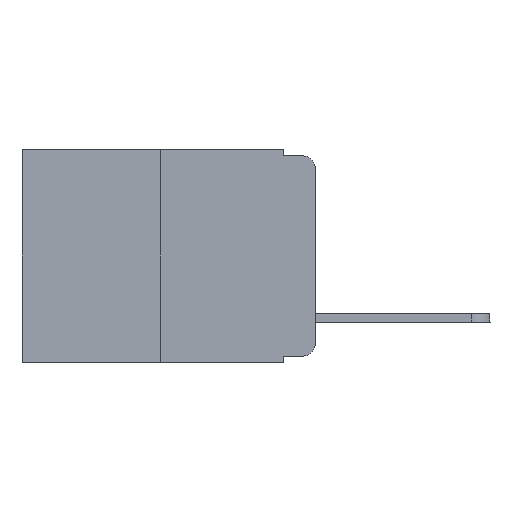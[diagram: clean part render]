
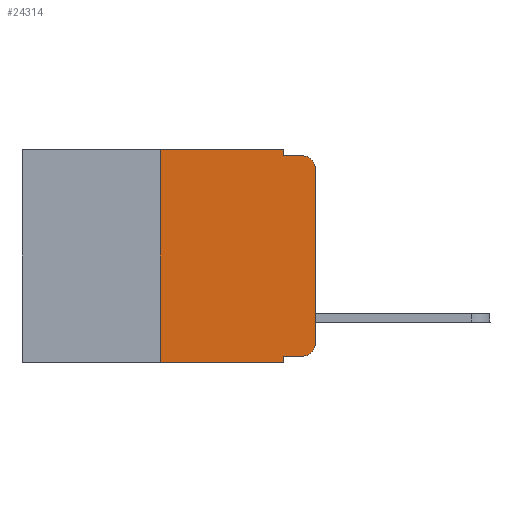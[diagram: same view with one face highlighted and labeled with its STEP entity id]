
A CAD part, left-side view. The second image highlights one B-rep face of the part: STEP entity #24314.
In plain terms, the highlighted planar face has unit normal (-1, 0, 0).
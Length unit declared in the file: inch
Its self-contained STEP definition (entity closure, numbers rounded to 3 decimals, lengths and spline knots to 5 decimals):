
#302 = VECTOR ( 'NONE', #13397, 39.37008 ) ;
#645 = CARTESIAN_POINT ( 'NONE',  ( 0., 0.473, 0. ) ) ;
#865 = ORIENTED_EDGE ( 'NONE', *, *, #11124, .T. ) ;
#1724 = DIRECTION ( 'NONE',  ( -1., 0., 0. ) ) ;
#1776 = VERTEX_POINT ( 'NONE', #15486 ) ;
#2022 = EDGE_CURVE ( 'NONE', #14431, #3511, #22727, .T. ) ;
#2153 = AXIS2_PLACEMENT_3D ( 'NONE', #15584, #1724, #21444 ) ;
#2289 = DIRECTION ( 'NONE',  ( 0., 0., -1. ) ) ;
#2413 = CARTESIAN_POINT ( 'NONE',  ( 0., 0., -0.03 ) ) ;
#2669 = EDGE_CURVE ( 'NONE', #3511, #21373, #8238, .T. ) ;
#3124 = EDGE_CURVE ( 'NONE', #24070, #15990, #22677, .T. ) ;
#3193 = CARTESIAN_POINT ( 'NONE',  ( 0., 0.051, 0. ) ) ;
#3511 = VERTEX_POINT ( 'NONE', #5101 ) ;
#3646 = LINE ( 'NONE', #9644, #7637 ) ;
#3664 = CIRCLE ( 'NONE', #4204, 0.02 ) ;
#3833 = VECTOR ( 'NONE', #7618, 39.37008 ) ;
#4204 = AXIS2_PLACEMENT_3D ( 'NONE', #8919, #16780, #22647 ) ;
#5101 = CARTESIAN_POINT ( 'NONE',  ( 0., 0.051, -0.01 ) ) ;
#5579 = ORIENTED_EDGE ( 'NONE', *, *, #6956, .F. ) ;
#6323 = VECTOR ( 'NONE', #7011, 39.37008 ) ;
#6493 = DIRECTION ( 'NONE',  ( 0., -1., 0. ) ) ;
#6956 = EDGE_CURVE ( 'NONE', #12416, #1776, #3646, .T. ) ;
#7011 = DIRECTION ( 'NONE',  ( 0., 0., 1. ) ) ;
#7618 = DIRECTION ( 'NONE',  ( 0., 0., -1. ) ) ;
#7637 = VECTOR ( 'NONE', #7837, 39.37008 ) ;
#7803 = DIRECTION ( 'NONE',  ( 1., 0., 0. ) ) ;
#7837 = DIRECTION ( 'NONE',  ( 0., 0., 1. ) ) ;
#8234 = ORIENTED_EDGE ( 'NONE', *, *, #22023, .T. ) ;
#8238 = LINE ( 'NONE', #8549, #23303 ) ;
#8549 = CARTESIAN_POINT ( 'NONE',  ( 0., 0.051, -0.01 ) ) ;
#8795 = DIRECTION ( 'NONE',  ( 0., -1., 0. ) ) ;
#8837 = ORIENTED_EDGE ( 'NONE', *, *, #18282, .F. ) ;
#8919 = CARTESIAN_POINT ( 'NONE',  ( 0., 0.02, -0.313 ) ) ;
#8943 = EDGE_CURVE ( 'NONE', #12416, #23056, #22262, .T. ) ;
#9061 = EDGE_CURVE ( 'NONE', #11862, #21373, #18533, .T. ) ;
#9142 = VECTOR ( 'NONE', #20288, 39.37008 ) ;
#9644 = CARTESIAN_POINT ( 'NONE',  ( 0., 0.25, 0. ) ) ;
#10115 = VECTOR ( 'NONE', #19527, 39.37008 ) ;
#10370 = ORIENTED_EDGE ( 'NONE', *, *, #9061, .T. ) ;
#10870 = CARTESIAN_POINT ( 'NONE',  ( 0., 0., -0.313 ) ) ;
#10943 = CARTESIAN_POINT ( 'NONE',  ( 0., 0.02, -0.01 ) ) ;
#11074 = ORIENTED_EDGE ( 'NONE', *, *, #3124, .T. ) ;
#11124 = EDGE_CURVE ( 'NONE', #13988, #11862, #11233, .T. ) ;
#11233 = LINE ( 'NONE', #13141, #6323 ) ;
#11252 = EDGE_LOOP ( 'NONE', ( #865, #10370, #16559, #22259, #22219, #5579, #21083, #8837, #11074, #8234 ) ) ;
#11862 = VERTEX_POINT ( 'NONE', #2413 ) ;
#11978 = CARTESIAN_POINT ( 'NONE',  ( 0., 0.051, -0.333 ) ) ;
#12416 = VERTEX_POINT ( 'NONE', #20490 ) ;
#13016 = VECTOR ( 'NONE', #6493, 39.37008 ) ;
#13141 = CARTESIAN_POINT ( 'NONE',  ( 0., 0., 0. ) ) ;
#13397 = DIRECTION ( 'NONE',  ( 0., 0., -1. ) ) ;
#13988 = VERTEX_POINT ( 'NONE', #10870 ) ;
#14431 = VERTEX_POINT ( 'NONE', #3193 ) ;
#14931 = LINE ( 'NONE', #645, #9142 ) ;
#15486 = CARTESIAN_POINT ( 'NONE',  ( 0., 0.25, 0. ) ) ;
#15584 = CARTESIAN_POINT ( 'NONE',  ( 0., 0.02, -0.03 ) ) ;
#15589 = EDGE_CURVE ( 'NONE', #1776, #14431, #14931, .T. ) ;
#15727 = CARTESIAN_POINT ( 'NONE',  ( 0., 0.051, 0. ) ) ;
#15990 = VERTEX_POINT ( 'NONE', #17557 ) ;
#16559 = ORIENTED_EDGE ( 'NONE', *, *, #2669, .F. ) ;
#16780 = DIRECTION ( 'NONE',  ( -1., 0., 0. ) ) ;
#17092 = CARTESIAN_POINT ( 'NONE',  ( 0., 0.051, -0.343 ) ) ;
#17459 = FACE_OUTER_BOUND ( 'NONE', #11252, .T. ) ;
#17555 = PLANE ( 'NONE',  #24443 ) ;
#17557 = CARTESIAN_POINT ( 'NONE',  ( 0., 0.02, -0.333 ) ) ;
#18282 = EDGE_CURVE ( 'NONE', #24070, #23056, #19469, .T. ) ;
#18533 = CIRCLE ( 'NONE', #2153, 0.02 ) ;
#19469 = LINE ( 'NONE', #15727, #3833 ) ;
#19527 = DIRECTION ( 'NONE',  ( 0., -1., 0. ) ) ;
#19541 = CARTESIAN_POINT ( 'NONE',  ( 0., 0.473, 0. ) ) ;
#20288 = DIRECTION ( 'NONE',  ( 0., -1., 0. ) ) ;
#20490 = CARTESIAN_POINT ( 'NONE',  ( 0., 0.25, -0.343 ) ) ;
#21083 = ORIENTED_EDGE ( 'NONE', *, *, #8943, .T. ) ;
#21215 = CARTESIAN_POINT ( 'NONE',  ( 0., 0.051, 0. ) ) ;
#21373 = VERTEX_POINT ( 'NONE', #10943 ) ;
#21444 = DIRECTION ( 'NONE',  ( 0., 0., -1. ) ) ;
#22011 = CARTESIAN_POINT ( 'NONE',  ( 0., 0.473, -0.343 ) ) ;
#22023 = EDGE_CURVE ( 'NONE', #15990, #13988, #3664, .T. ) ;
#22219 = ORIENTED_EDGE ( 'NONE', *, *, #15589, .F. ) ;
#22259 = ORIENTED_EDGE ( 'NONE', *, *, #2022, .F. ) ;
#22262 = LINE ( 'NONE', #22011, #13016 ) ;
#22319 = CARTESIAN_POINT ( 'NONE',  ( 0., 0.051, -0.333 ) ) ;
#22647 = DIRECTION ( 'NONE',  ( 0., 0., -1. ) ) ;
#22677 = LINE ( 'NONE', #11978, #10115 ) ;
#22727 = LINE ( 'NONE', #21215, #302 ) ;
#23056 = VERTEX_POINT ( 'NONE', #17092 ) ;
#23303 = VECTOR ( 'NONE', #8795, 39.37008 ) ;
#24070 = VERTEX_POINT ( 'NONE', #22319 ) ;
#24314 = ADVANCED_FACE ( 'NONE', ( #17459 ), #17555, .F. ) ;
#24443 = AXIS2_PLACEMENT_3D ( 'NONE', #19541, #7803, #2289 ) ;
